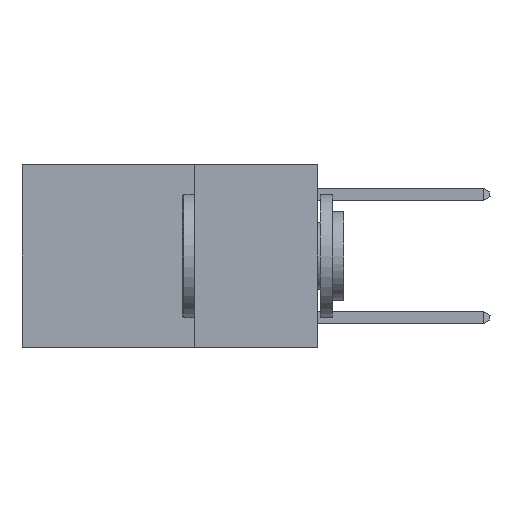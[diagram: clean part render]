
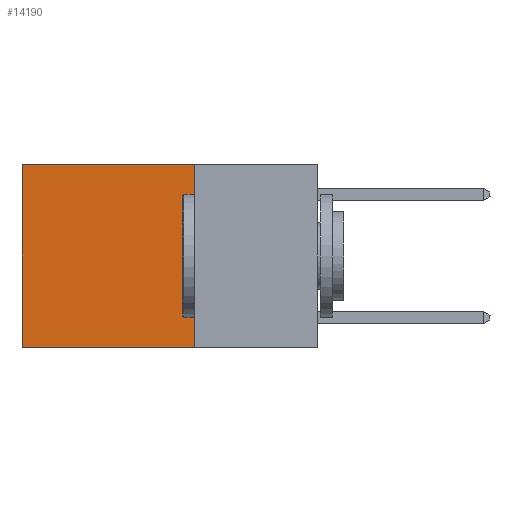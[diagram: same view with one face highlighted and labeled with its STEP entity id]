
A CAD part, left-side view. The second image highlights one B-rep face of the part: STEP entity #14190.
In plain terms, the highlighted planar face has unit normal (-1, 0, 0).
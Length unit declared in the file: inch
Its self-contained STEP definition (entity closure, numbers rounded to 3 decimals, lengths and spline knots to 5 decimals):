
#454 = CARTESIAN_POINT ( 'NONE',  ( 0.2625, 0.25, -0.37 ) ) ;
#925 = VECTOR ( 'NONE', #11484, 39.37008 ) ;
#1117 = LINE ( 'NONE', #10701, #5530 ) ;
#1397 = ORIENTED_EDGE ( 'NONE', *, *, #3689, .F. ) ;
#1456 = VERTEX_POINT ( 'NONE', #454 ) ;
#3396 = EDGE_CURVE ( 'NONE', #13416, #4474, #16462, .T. ) ;
#3410 = VERTEX_POINT ( 'NONE', #10173 ) ;
#3632 = CARTESIAN_POINT ( 'NONE',  ( 0.2625, 0.6, 0. ) ) ;
#3689 = EDGE_CURVE ( 'NONE', #13416, #1456, #1117, .T. ) ;
#3942 = DIRECTION ( 'NONE',  ( 1., 0., 0. ) ) ;
#4179 = DIRECTION ( 'NONE',  ( 0., 1., 0. ) ) ;
#4474 = VERTEX_POINT ( 'NONE', #13529 ) ;
#5067 = VECTOR ( 'NONE', #6191, 39.37008 ) ;
#5128 = CARTESIAN_POINT ( 'NONE',  ( 0.2625, 0.25, 0. ) ) ;
#5530 = VECTOR ( 'NONE', #9500, 39.37008 ) ;
#6191 = DIRECTION ( 'NONE',  ( 0., 0., -1. ) ) ;
#6455 = ORIENTED_EDGE ( 'NONE', *, *, #8508, .T. ) ;
#7181 = AXIS2_PLACEMENT_3D ( 'NONE', #14513, #3942, #12999 ) ;
#7615 = ORIENTED_EDGE ( 'NONE', *, *, #10719, .F. ) ;
#8508 = EDGE_CURVE ( 'NONE', #4474, #3410, #16600, .T. ) ;
#9500 = DIRECTION ( 'NONE',  ( 0., 0., -1. ) ) ;
#10018 = ORIENTED_EDGE ( 'NONE', *, *, #3396, .T. ) ;
#10173 = CARTESIAN_POINT ( 'NONE',  ( 0.2625, 0.6, -0.37 ) ) ;
#10234 = FACE_OUTER_BOUND ( 'NONE', #12385, .T. ) ;
#10434 = CARTESIAN_POINT ( 'NONE',  ( 0.2625, 0.25, 0. ) ) ;
#10701 = CARTESIAN_POINT ( 'NONE',  ( 0.2625, 0.25, 0. ) ) ;
#10719 = EDGE_CURVE ( 'NONE', #1456, #3410, #10795, .T. ) ;
#10795 = LINE ( 'NONE', #11945, #11263 ) ;
#11263 = VECTOR ( 'NONE', #4179, 39.37008 ) ;
#11484 = DIRECTION ( 'NONE',  ( 0., 1., 0. ) ) ;
#11945 = CARTESIAN_POINT ( 'NONE',  ( 0.2625, 0.25, -0.37 ) ) ;
#12385 = EDGE_LOOP ( 'NONE', ( #6455, #7615, #1397, #10018 ) ) ;
#12999 = DIRECTION ( 'NONE',  ( 0., 0., -1. ) ) ;
#13228 = PLANE ( 'NONE',  #7181 ) ;
#13416 = VERTEX_POINT ( 'NONE', #10434 ) ;
#13529 = CARTESIAN_POINT ( 'NONE',  ( 0.2625, 0.6, 0. ) ) ;
#14190 = ADVANCED_FACE ( 'NONE', ( #10234 ), #13228, .F. ) ;
#14513 = CARTESIAN_POINT ( 'NONE',  ( 0.2625, 0.25, 0. ) ) ;
#16462 = LINE ( 'NONE', #5128, #925 ) ;
#16600 = LINE ( 'NONE', #3632, #5067 ) ;
